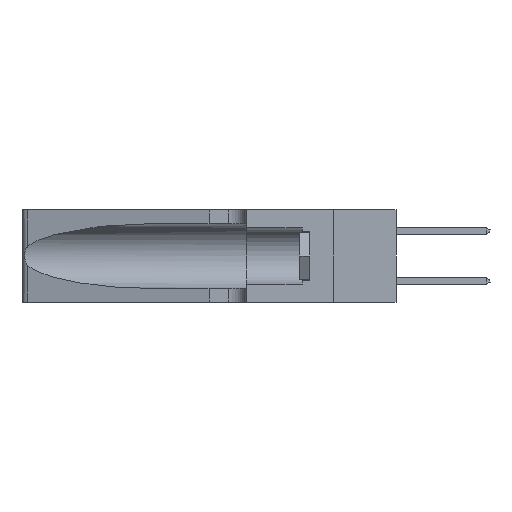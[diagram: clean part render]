
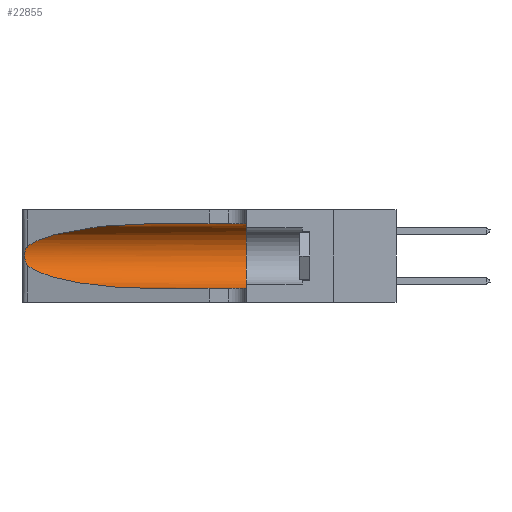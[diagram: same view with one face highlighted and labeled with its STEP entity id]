
A CAD part, left-side view. The second image highlights one B-rep face of the part: STEP entity #22855.
In plain terms, the highlighted cylindrical face has radius 3.308 mm (diameter 6.617 mm), a partial arc.
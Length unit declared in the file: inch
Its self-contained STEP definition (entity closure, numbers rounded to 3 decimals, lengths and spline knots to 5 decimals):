
#67 = CARTESIAN_POINT ( 'NONE',  ( 0.25487, 1.22718, 0.14631 ) ) ;
#145 = B_SPLINE_CURVE_WITH_KNOTS ( 'NONE', 3,
 ( #265, #15530, #23066, #7998, #25525, #10537, #27997, #13110, #30502, #15642, #371, #18152, #2999, #20678 ),
 .UNSPECIFIED., .F., .F.,
 ( 4, 2, 2, 2, 2, 2, 4 ),
 ( 0., 0.00027, 0.00053, 0.00107, 0.0016, 0.00187, 0.00214 ),
 .UNSPECIFIED. ) ;
#173 = CARTESIAN_POINT ( 'NONE',  ( 0.1305, 0.72297, 0.31525 ) ) ;
#265 = CARTESIAN_POINT ( 'NONE',  ( 0.25487, 1.22718, 0.22369 ) ) ;
#371 = CARTESIAN_POINT ( 'NONE',  ( 0.25789, 1.23486, 0.15765 ) ) ;
#1121 = CARTESIAN_POINT ( 'NONE',  ( 0.25487, 1.22718, 0.22369 ) ) ;
#1259 = CARTESIAN_POINT ( 'NONE',  ( 0.1305, 1.61858, 0.185 ) ) ;
#1327 = VECTOR ( 'NONE', #2603, 39.37008 ) ;
#1512 = VERTEX_POINT ( 'NONE', #11540 ) ;
#1529 =( BOUNDED_CURVE ( )  B_SPLINE_CURVE ( 3, ( #28682, #11271, #16355, #1121 ),
 .UNSPECIFIED., .F., .F. ) 
 B_SPLINE_CURVE_WITH_KNOTS ( ( 4, 4 ),
 ( 1.5708, 2.84003 ),
 .UNSPECIFIED. ) 
 CURVE ( )  GEOMETRIC_REPRESENTATION_ITEM ( )  RATIONAL_B_SPLINE_CURVE ( ( 1., 0.87, 0.87, 1. ) ) 
 REPRESENTATION_ITEM ( '' )  );
#1852 = VERTEX_POINT ( 'NONE', #18557 ) ;
#2415 = ORIENTED_EDGE ( 'NONE', *, *, #20414, .F. ) ;
#2603 = DIRECTION ( 'NONE',  ( 0., -1., 0. ) ) ;
#2999 = CARTESIAN_POINT ( 'NONE',  ( 0.25555, 1.22993, 0.14849 ) ) ;
#3003 = ORIENTED_EDGE ( 'NONE', *, *, #26580, .T. ) ;
#4021 = CIRCLE ( 'NONE', #9983, 0.13025 ) ;
#4311 = VERTEX_POINT ( 'NONE', #25268 ) ;
#4360 = CARTESIAN_POINT ( 'NONE',  ( 0.1305, 0.35, 0.185 ) ) ;
#4977 = CARTESIAN_POINT ( 'NONE',  ( 0.1305, 0.35, 0.31525 ) ) ;
#5113 = EDGE_CURVE ( 'NONE', #16968, #28804, #22680, .T. ) ;
#5300 = CARTESIAN_POINT ( 'NONE',  ( 0.18966, 0.96281, 0.05475 ) ) ;
#6466 = ORIENTED_EDGE ( 'NONE', *, *, #30370, .T. ) ;
#6920 = DIRECTION ( 'NONE',  ( 0., 0., 1. ) ) ;
#7998 = CARTESIAN_POINT ( 'NONE',  ( 0.25787, 1.23484, 0.2124 ) ) ;
#8212 = EDGE_LOOP ( 'NONE', ( #3003, #30095, #14454, #6466, #2415, #14096 ) ) ;
#8954 = DIRECTION ( 'NONE',  ( 0., 0., -1. ) ) ;
#9679 = VERTEX_POINT ( 'NONE', #12671 ) ;
#9701 = LINE ( 'NONE', #12624, #1327 ) ;
#9983 = AXIS2_PLACEMENT_3D ( 'NONE', #4360, #21969, #6920 ) ;
#10537 = CARTESIAN_POINT ( 'NONE',  ( 0.26018, 1.23835, 0.19895 ) ) ;
#11271 = CARTESIAN_POINT ( 'NONE',  ( 0.18966, 0.96281, 0.31525 ) ) ;
#11540 = CARTESIAN_POINT ( 'NONE',  ( 0.1305, 0.35, 0.05475 ) ) ;
#12624 = CARTESIAN_POINT ( 'NONE',  ( 0.1305, 1.61858, 0.05475 ) ) ;
#12671 = CARTESIAN_POINT ( 'NONE',  ( 0.25487, 1.22718, 0.22369 ) ) ;
#13110 = CARTESIAN_POINT ( 'NONE',  ( 0.26075, 1.23896, 0.178 ) ) ;
#13349 =( BOUNDED_CURVE ( )  B_SPLINE_CURVE ( 3, ( #67, #15352, #5300, #22876 ),
 .UNSPECIFIED., .F., .F. ) 
 B_SPLINE_CURVE_WITH_KNOTS ( ( 4, 4 ),
 ( 3.44316, 4.71239 ),
 .UNSPECIFIED. ) 
 CURVE ( )  GEOMETRIC_REPRESENTATION_ITEM ( )  RATIONAL_B_SPLINE_CURVE ( ( 1., 0.87, 0.87, 1. ) ) 
 REPRESENTATION_ITEM ( '' )  );
#13548 = CARTESIAN_POINT ( 'NONE',  ( 0.1305, 1.61858, 0.31525 ) ) ;
#13947 = DIRECTION ( 'NONE',  ( 0., -1., 0. ) ) ;
#14096 = ORIENTED_EDGE ( 'NONE', *, *, #5113, .F. ) ;
#14454 = ORIENTED_EDGE ( 'NONE', *, *, #23554, .T. ) ;
#15352 = CARTESIAN_POINT ( 'NONE',  ( 0.2373, 1.15595, 0.08982 ) ) ;
#15530 = CARTESIAN_POINT ( 'NONE',  ( 0.25555, 1.22994, 0.2215 ) ) ;
#15642 = CARTESIAN_POINT ( 'NONE',  ( 0.25856, 1.23593, 0.16098 ) ) ;
#16045 = VECTOR ( 'NONE', #28420, 39.37008 ) ;
#16355 = CARTESIAN_POINT ( 'NONE',  ( 0.2373, 1.15595, 0.28018 ) ) ;
#16968 = VERTEX_POINT ( 'NONE', #173 ) ;
#17445 = AXIS2_PLACEMENT_3D ( 'NONE', #1259, #13947, #8954 ) ;
#18152 = CARTESIAN_POINT ( 'NONE',  ( 0.25639, 1.23186, 0.15144 ) ) ;
#18557 = CARTESIAN_POINT ( 'NONE',  ( 0.1305, 0.72297, 0.05475 ) ) ;
#20414 = EDGE_CURVE ( 'NONE', #28804, #1512, #4021, .T. ) ;
#20678 = CARTESIAN_POINT ( 'NONE',  ( 0.25487, 1.22718, 0.14631 ) ) ;
#21969 = DIRECTION ( 'NONE',  ( 0., 1., 0. ) ) ;
#22049 = EDGE_CURVE ( 'NONE', #9679, #4311, #145, .T. ) ;
#22395 = FACE_OUTER_BOUND ( 'NONE', #8212, .T. ) ;
#22680 = LINE ( 'NONE', #13548, #16045 ) ;
#22855 = ADVANCED_FACE ( 'NONE', ( #22395 ), #28172, .F. ) ;
#22876 = CARTESIAN_POINT ( 'NONE',  ( 0.1305, 0.72297, 0.05475 ) ) ;
#23066 = CARTESIAN_POINT ( 'NONE',  ( 0.25639, 1.23184, 0.21858 ) ) ;
#23554 = EDGE_CURVE ( 'NONE', #4311, #1852, #13349, .T. ) ;
#25268 = CARTESIAN_POINT ( 'NONE',  ( 0.25487, 1.22718, 0.14631 ) ) ;
#25525 = CARTESIAN_POINT ( 'NONE',  ( 0.25854, 1.2359, 0.20912 ) ) ;
#26580 = EDGE_CURVE ( 'NONE', #16968, #9679, #1529, .T. ) ;
#27997 = CARTESIAN_POINT ( 'NONE',  ( 0.26075, 1.23896, 0.19203 ) ) ;
#28172 = CYLINDRICAL_SURFACE ( 'NONE', #17445, 0.13025 ) ;
#28420 = DIRECTION ( 'NONE',  ( 0., -1., 0. ) ) ;
#28682 = CARTESIAN_POINT ( 'NONE',  ( 0.1305, 0.72297, 0.31525 ) ) ;
#28804 = VERTEX_POINT ( 'NONE', #4977 ) ;
#30095 = ORIENTED_EDGE ( 'NONE', *, *, #22049, .T. ) ;
#30370 = EDGE_CURVE ( 'NONE', #1852, #1512, #9701, .T. ) ;
#30502 = CARTESIAN_POINT ( 'NONE',  ( 0.26017, 1.23833, 0.17102 ) ) ;
